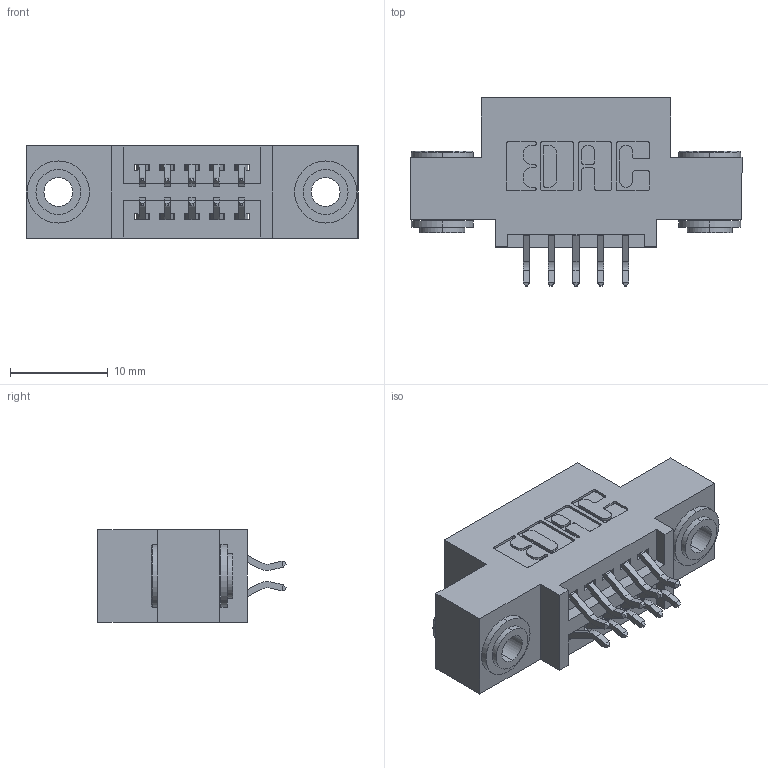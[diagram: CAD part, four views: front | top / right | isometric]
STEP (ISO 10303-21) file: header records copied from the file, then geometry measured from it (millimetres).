
FILE_DESCRIPTION (( 'STEP AP203' ), '1' );
FILE_NAME ('345-010-556-503.STEP', '2019-10-26T14:46:53', ( '' ), ( '' ), 'SwSTEP 2.0', 'SolidWorks 2016', '' );
FILE_SCHEMA (( 'CONFIG_CONTROL_DESIGN' ));
Length unit declared in the file: inch
Products named in the file (4): 345-292-001_556 Tail; 345-010-556-503; 345 Part_0.110 Offset - 0.156 Dia-TH; 345-250-002_345-250-002-102
Assembly tree (13 placements, depth 2):
  345-010-556-503
    345 Part_0.110 Offset - 0.156 Dia-TH
    345-292-001_556 Tail  x10
    345-250-002_345-250-002-102  x2
Bounding box: 33.91 x 19.24 x 9.4 mm (x, y, z)
Volume: 2896.1 mm3; surface area: 3853.3 mm2
Topology: 13 solids, 13 shells, 728 faces, 2099 edges, 1382 vertices
Faces by surface type: plane 464, cylinder 256, cone 8
Entity records: 9906 total; most frequent: CARTESIAN_POINT 1687, ORIENTED_EDGE 1602, DIRECTION 1551, EDGE_CURVE 801, VECTOR 617, LINE 617, VERTEX_POINT 530, AXIS2_PLACEMENT_3D 467
